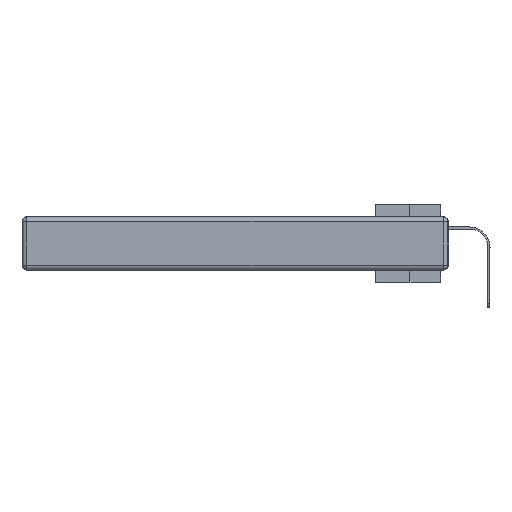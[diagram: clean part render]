
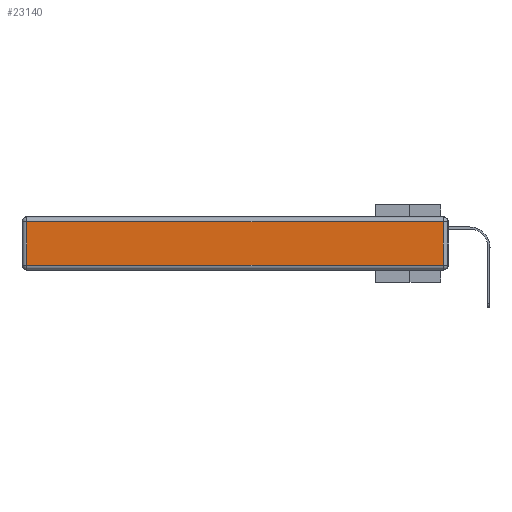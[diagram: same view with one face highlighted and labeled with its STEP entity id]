
A CAD part, left-side view. The second image highlights one B-rep face of the part: STEP entity #23140.
In plain terms, the highlighted planar face has unit normal (-1, 0, 0).
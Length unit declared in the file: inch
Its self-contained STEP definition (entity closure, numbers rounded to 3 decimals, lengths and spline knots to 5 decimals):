
#1428 = ORIENTED_EDGE ( 'NONE', *, *, #26379, .T. ) ;
#2755 = DIRECTION ( 'NONE',  ( -1., 0., 0. ) ) ;
#4155 = CARTESIAN_POINT ( 'NONE',  ( 0., 0., -0.313 ) ) ;
#4939 = ORIENTED_EDGE ( 'NONE', *, *, #31056, .T. ) ;
#5603 = LINE ( 'NONE', #15315, #8378 ) ;
#6343 = DIRECTION ( 'NONE',  ( 0., 0., -1. ) ) ;
#6873 = CARTESIAN_POINT ( 'NONE',  ( 0., 2.72, -0.03 ) ) ;
#7796 = AXIS2_PLACEMENT_3D ( 'NONE', #9961, #2755, #15335 ) ;
#8378 = VECTOR ( 'NONE', #15483, 39.37008 ) ;
#8550 = EDGE_CURVE ( 'NONE', #12727, #27235, #5603, .T. ) ;
#8622 = VECTOR ( 'NONE', #24256, 39.37008 ) ;
#9961 = CARTESIAN_POINT ( 'NONE',  ( 0., 0., -0.343 ) ) ;
#10808 = LINE ( 'NONE', #25645, #27747 ) ;
#11261 = VERTEX_POINT ( 'NONE', #18902 ) ;
#12117 = LINE ( 'NONE', #24084, #30179 ) ;
#12727 = VERTEX_POINT ( 'NONE', #30193 ) ;
#14654 = DIRECTION ( 'NONE',  ( 0., 1., 0. ) ) ;
#14728 = EDGE_CURVE ( 'NONE', #26447, #11261, #10808, .T. ) ;
#15315 = CARTESIAN_POINT ( 'NONE',  ( 0., 0.03, -0.343 ) ) ;
#15335 = DIRECTION ( 'NONE',  ( 0., 0., 1. ) ) ;
#15483 = DIRECTION ( 'NONE',  ( 0., 0., 1. ) ) ;
#16729 = EDGE_LOOP ( 'NONE', ( #1428, #28204, #4939, #27698 ) ) ;
#18902 = CARTESIAN_POINT ( 'NONE',  ( 0., 2.72, -0.313 ) ) ;
#21069 = LINE ( 'NONE', #4155, #8622 ) ;
#22367 = CARTESIAN_POINT ( 'NONE',  ( 0., 0.03, -0.03 ) ) ;
#23140 = ADVANCED_FACE ( 'NONE', ( #27015 ), #24622, .T. ) ;
#24084 = CARTESIAN_POINT ( 'NONE',  ( 0., 2.75, -0.03 ) ) ;
#24256 = DIRECTION ( 'NONE',  ( 0., -1., 0. ) ) ;
#24622 = PLANE ( 'NONE',  #7796 ) ;
#25645 = CARTESIAN_POINT ( 'NONE',  ( 0., 2.72, -0.343 ) ) ;
#26379 = EDGE_CURVE ( 'NONE', #11261, #12727, #21069, .T. ) ;
#26447 = VERTEX_POINT ( 'NONE', #6873 ) ;
#27015 = FACE_OUTER_BOUND ( 'NONE', #16729, .T. ) ;
#27235 = VERTEX_POINT ( 'NONE', #22367 ) ;
#27698 = ORIENTED_EDGE ( 'NONE', *, *, #14728, .T. ) ;
#27747 = VECTOR ( 'NONE', #6343, 39.37008 ) ;
#28204 = ORIENTED_EDGE ( 'NONE', *, *, #8550, .T. ) ;
#30179 = VECTOR ( 'NONE', #14654, 39.37008 ) ;
#30193 = CARTESIAN_POINT ( 'NONE',  ( 0., 0.03, -0.313 ) ) ;
#31056 = EDGE_CURVE ( 'NONE', #27235, #26447, #12117, .T. ) ;
